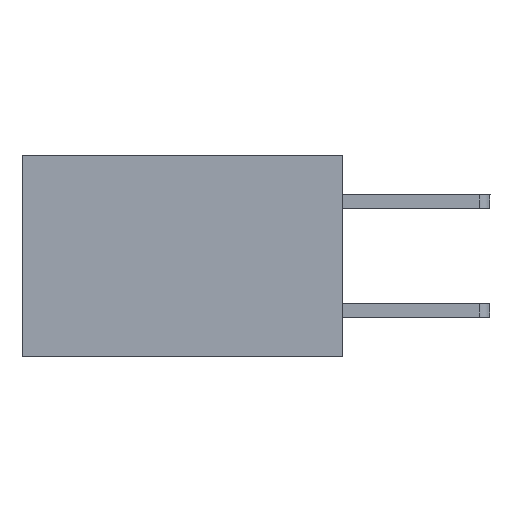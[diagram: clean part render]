
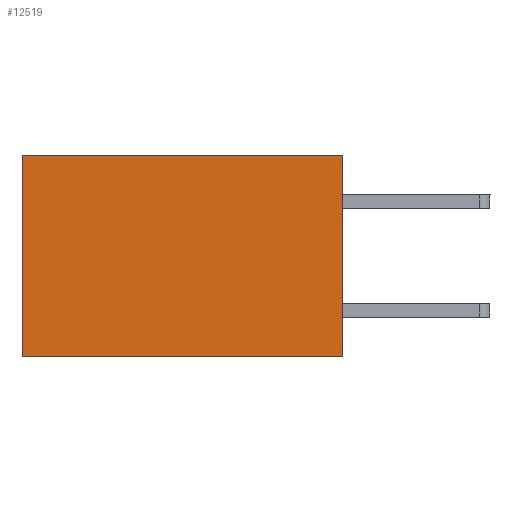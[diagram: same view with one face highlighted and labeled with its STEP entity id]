
A CAD part, left-side view. The second image highlights one B-rep face of the part: STEP entity #12519.
In plain terms, the highlighted planar face has unit normal (-1, 0, 0).
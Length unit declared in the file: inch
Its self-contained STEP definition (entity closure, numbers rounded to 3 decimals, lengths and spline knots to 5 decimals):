
#499 = EDGE_CURVE ( 'NONE', #8854, #2400, #10192, .T. ) ;
#839 = PLANE ( 'NONE',  #2582 ) ;
#1829 = LINE ( 'NONE', #3625, #9030 ) ;
#2155 = DIRECTION ( 'NONE',  ( 0., 0., -1. ) ) ;
#2400 = VERTEX_POINT ( 'NONE', #5182 ) ;
#2582 = AXIS2_PLACEMENT_3D ( 'NONE', #12804, #9837, #11807 ) ;
#2968 = ORIENTED_EDGE ( 'NONE', *, *, #5623, .F. ) ;
#2999 = CARTESIAN_POINT ( 'NONE',  ( 0.277, 0., 0. ) ) ;
#3035 = LINE ( 'NONE', #12263, #11544 ) ;
#3625 = CARTESIAN_POINT ( 'NONE',  ( 0.277, 0., -0.37 ) ) ;
#3761 = CARTESIAN_POINT ( 'NONE',  ( 0.277, 0.59, -0.37 ) ) ;
#4061 = LINE ( 'NONE', #12220, #9247 ) ;
#4073 = DIRECTION ( 'NONE',  ( 0., 1., 0. ) ) ;
#4771 = ORIENTED_EDGE ( 'NONE', *, *, #499, .T. ) ;
#4932 = EDGE_LOOP ( 'NONE', ( #11561, #5663, #2968, #4771 ) ) ;
#5182 = CARTESIAN_POINT ( 'NONE',  ( 0.277, 0.59, 0. ) ) ;
#5593 = VERTEX_POINT ( 'NONE', #12524 ) ;
#5623 = EDGE_CURVE ( 'NONE', #8854, #5593, #4061, .T. ) ;
#5663 = ORIENTED_EDGE ( 'NONE', *, *, #12884, .F. ) ;
#6532 = DIRECTION ( 'NONE',  ( 0., 0., -1. ) ) ;
#7111 = VERTEX_POINT ( 'NONE', #3761 ) ;
#8387 = CARTESIAN_POINT ( 'NONE',  ( 0.277, 0., 0. ) ) ;
#8854 = VERTEX_POINT ( 'NONE', #8387 ) ;
#9030 = VECTOR ( 'NONE', #11855, 39.37008 ) ;
#9247 = VECTOR ( 'NONE', #6532, 39.37008 ) ;
#9837 = DIRECTION ( 'NONE',  ( 1., 0., 0. ) ) ;
#10192 = LINE ( 'NONE', #2999, #12453 ) ;
#11544 = VECTOR ( 'NONE', #2155, 39.37008 ) ;
#11561 = ORIENTED_EDGE ( 'NONE', *, *, #12609, .T. ) ;
#11807 = DIRECTION ( 'NONE',  ( 0., 0., -1. ) ) ;
#11855 = DIRECTION ( 'NONE',  ( 0., 1., 0. ) ) ;
#12220 = CARTESIAN_POINT ( 'NONE',  ( 0.277, 0., -0.37 ) ) ;
#12263 = CARTESIAN_POINT ( 'NONE',  ( 0.277, 0.59, -0.37 ) ) ;
#12453 = VECTOR ( 'NONE', #4073, 39.37008 ) ;
#12519 = ADVANCED_FACE ( 'NONE', ( #13006 ), #839, .F. ) ;
#12524 = CARTESIAN_POINT ( 'NONE',  ( 0.277, 0., -0.37 ) ) ;
#12609 = EDGE_CURVE ( 'NONE', #2400, #7111, #3035, .T. ) ;
#12804 = CARTESIAN_POINT ( 'NONE',  ( 0.277, 0., -0.37 ) ) ;
#12884 = EDGE_CURVE ( 'NONE', #5593, #7111, #1829, .T. ) ;
#13006 = FACE_OUTER_BOUND ( 'NONE', #4932, .T. ) ;
